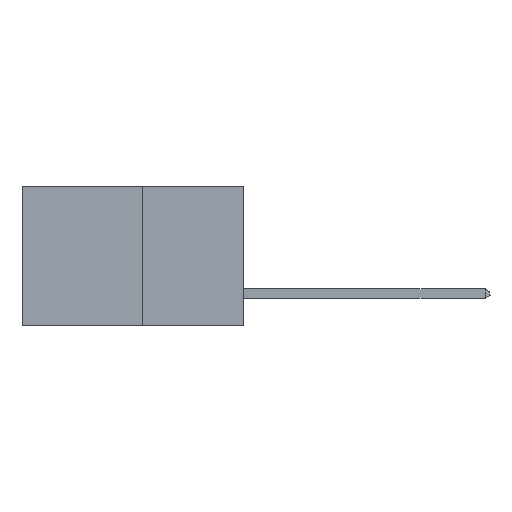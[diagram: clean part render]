
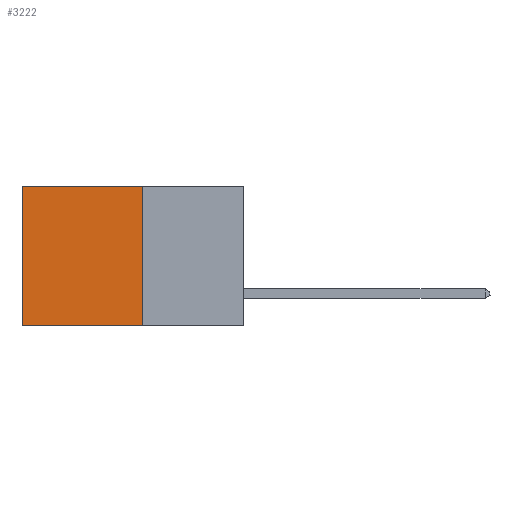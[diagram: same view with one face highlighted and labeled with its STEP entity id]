
A CAD part, left-side view. The second image highlights one B-rep face of the part: STEP entity #3222.
In plain terms, the highlighted planar face has unit normal (-1, 0, 0).
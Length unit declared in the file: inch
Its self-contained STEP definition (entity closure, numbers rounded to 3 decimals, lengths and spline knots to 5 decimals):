
#480 = DIRECTION ( 'NONE',  ( 1., 0., 0. ) ) ;
#574 = EDGE_CURVE ( 'NONE', #1113, #2355, #10507, .T. ) ;
#645 = VERTEX_POINT ( 'NONE', #4936 ) ;
#699 = CARTESIAN_POINT ( 'NONE',  ( 0.277, 0.27, -0.37 ) ) ;
#1113 = VERTEX_POINT ( 'NONE', #6974 ) ;
#1299 = CARTESIAN_POINT ( 'NONE',  ( 0.277, 0.59, 0. ) ) ;
#1345 = EDGE_CURVE ( 'NONE', #2082, #2355, #10370, .T. ) ;
#2082 = VERTEX_POINT ( 'NONE', #1299 ) ;
#2108 = EDGE_CURVE ( 'NONE', #645, #2082, #5008, .T. ) ;
#2158 = VECTOR ( 'NONE', #6173, 39.37008 ) ;
#2355 = VERTEX_POINT ( 'NONE', #8254 ) ;
#2412 = ORIENTED_EDGE ( 'NONE', *, *, #6401, .F. ) ;
#2740 = VECTOR ( 'NONE', #6547, 39.37008 ) ;
#3092 = VECTOR ( 'NONE', #8179, 39.37008 ) ;
#3222 = ADVANCED_FACE ( 'NONE', ( #8708 ), #7150, .F. ) ;
#4118 = VECTOR ( 'NONE', #8724, 39.37008 ) ;
#4806 = CARTESIAN_POINT ( 'NONE',  ( 0.277, 0.27, -0.37 ) ) ;
#4936 = CARTESIAN_POINT ( 'NONE',  ( 0.277, 0.27, 0. ) ) ;
#4974 = ORIENTED_EDGE ( 'NONE', *, *, #2108, .T. ) ;
#5008 = LINE ( 'NONE', #7595, #2740 ) ;
#6173 = DIRECTION ( 'NONE',  ( 0., 0., -1. ) ) ;
#6210 = CARTESIAN_POINT ( 'NONE',  ( 0.277, 0.59, -0.37 ) ) ;
#6401 = EDGE_CURVE ( 'NONE', #645, #1113, #9425, .T. ) ;
#6547 = DIRECTION ( 'NONE',  ( 0., 1., 0. ) ) ;
#6605 = DIRECTION ( 'NONE',  ( 0., 0., -1. ) ) ;
#6974 = CARTESIAN_POINT ( 'NONE',  ( 0.277, 0.27, -0.37 ) ) ;
#7150 = PLANE ( 'NONE',  #9720 ) ;
#7396 = CARTESIAN_POINT ( 'NONE',  ( 0.277, 0.27, -0.37 ) ) ;
#7595 = CARTESIAN_POINT ( 'NONE',  ( 0.277, 0.27, 0. ) ) ;
#8179 = DIRECTION ( 'NONE',  ( 0., 0., -1. ) ) ;
#8254 = CARTESIAN_POINT ( 'NONE',  ( 0.277, 0.59, -0.37 ) ) ;
#8474 = EDGE_LOOP ( 'NONE', ( #9119, #10550, #2412, #4974 ) ) ;
#8708 = FACE_OUTER_BOUND ( 'NONE', #8474, .T. ) ;
#8724 = DIRECTION ( 'NONE',  ( 0., 1., 0. ) ) ;
#9119 = ORIENTED_EDGE ( 'NONE', *, *, #1345, .T. ) ;
#9425 = LINE ( 'NONE', #7396, #3092 ) ;
#9720 = AXIS2_PLACEMENT_3D ( 'NONE', #699, #480, #6605 ) ;
#10370 = LINE ( 'NONE', #6210, #2158 ) ;
#10507 = LINE ( 'NONE', #4806, #4118 ) ;
#10550 = ORIENTED_EDGE ( 'NONE', *, *, #574, .F. ) ;
